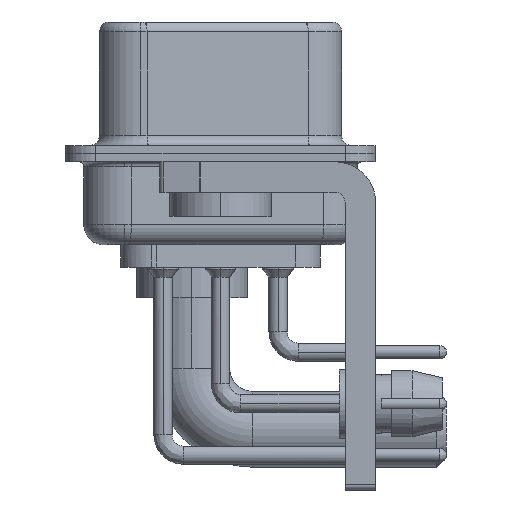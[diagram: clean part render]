
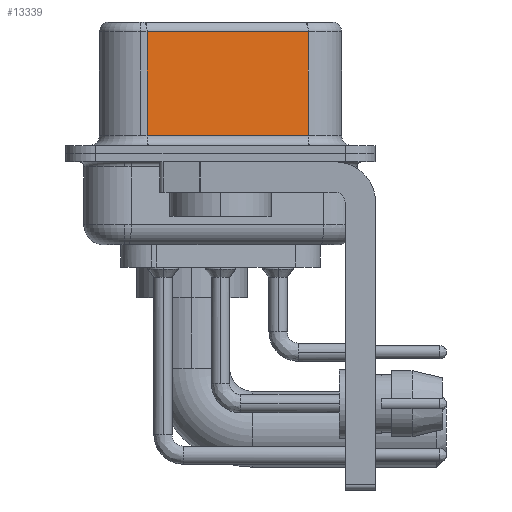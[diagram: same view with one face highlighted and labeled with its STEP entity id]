
A CAD part, left-side view. The second image highlights one B-rep face of the part: STEP entity #13339.
In plain terms, the highlighted planar face has unit normal (-0.985, -0.174, 0).
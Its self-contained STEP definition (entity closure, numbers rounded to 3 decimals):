
#404 = AXIS2_PLACEMENT_3D ( 'NONE', #25251, #5869, #31302 ) ;
#545 = PLANE ( 'NONE',  #404 ) ;
#2550 = CARTESIAN_POINT ( 'NONE',  ( 3.73, 3.628, 6.52 ) ) ;
#2779 = EDGE_LOOP ( 'NONE', ( #37489, #9758, #4748, #27221 ) ) ;
#4337 = EDGE_CURVE ( 'NONE', #12516, #39267, #35794, .T. ) ;
#4381 = LINE ( 'NONE', #7809, #28007 ) ;
#4582 = DIRECTION ( 'NONE',  ( 0.174, -0.985, 0. ) ) ;
#4748 = ORIENTED_EDGE ( 'NONE', *, *, #17851, .T. ) ;
#4954 = CARTESIAN_POINT ( 'NONE',  ( 3.73, 3.628, 6.02 ) ) ;
#5657 = LINE ( 'NONE', #23875, #7018 ) ;
#5869 = DIRECTION ( 'NONE',  ( 0.985, 0.174, 0. ) ) ;
#7018 = VECTOR ( 'NONE', #30346, 1000. ) ;
#7809 = CARTESIAN_POINT ( 'NONE',  ( 5.132, -4.322, 0.9 ) ) ;
#8096 = CARTESIAN_POINT ( 'NONE',  ( 5.132, -4.322, 6.02 ) ) ;
#9613 = VERTEX_POINT ( 'NONE', #18219 ) ;
#9758 = ORIENTED_EDGE ( 'NONE', *, *, #4337, .T. ) ;
#10350 = EDGE_CURVE ( 'NONE', #9613, #20329, #4381, .T. ) ;
#12516 = VERTEX_POINT ( 'NONE', #27430 ) ;
#13339 = ADVANCED_FACE ( 'NONE', ( #24087 ), #545, .F. ) ;
#16778 = EDGE_CURVE ( 'NONE', #12516, #20329, #5657, .T. ) ;
#17851 = EDGE_CURVE ( 'NONE', #39267, #9613, #33669, .T. ) ;
#18219 = CARTESIAN_POINT ( 'NONE',  ( 3.73, 3.628, 0.9 ) ) ;
#20017 = VECTOR ( 'NONE', #24595, 1000. ) ;
#20329 = VERTEX_POINT ( 'NONE', #22159 ) ;
#22159 = CARTESIAN_POINT ( 'NONE',  ( 5.132, -4.322, 0.9 ) ) ;
#23875 = CARTESIAN_POINT ( 'NONE',  ( 5.132, -4.322, 6.52 ) ) ;
#24087 = FACE_OUTER_BOUND ( 'NONE', #2779, .T. ) ;
#24595 = DIRECTION ( 'NONE',  ( 0., 0., -1. ) ) ;
#25251 = CARTESIAN_POINT ( 'NONE',  ( 5.132, -4.322, 6.52 ) ) ;
#27221 = ORIENTED_EDGE ( 'NONE', *, *, #10350, .T. ) ;
#27430 = CARTESIAN_POINT ( 'NONE',  ( 5.132, -4.322, 6.02 ) ) ;
#28007 = VECTOR ( 'NONE', #4582, 1000. ) ;
#30346 = DIRECTION ( 'NONE',  ( 0., 0., -1. ) ) ;
#31302 = DIRECTION ( 'NONE',  ( -0.174, 0.985, 0. ) ) ;
#33669 = LINE ( 'NONE', #2550, #20017 ) ;
#35168 = VECTOR ( 'NONE', #39045, 1000. ) ;
#35794 = LINE ( 'NONE', #8096, #35168 ) ;
#37489 = ORIENTED_EDGE ( 'NONE', *, *, #16778, .F. ) ;
#39045 = DIRECTION ( 'NONE',  ( -0.174, 0.985, 0. ) ) ;
#39267 = VERTEX_POINT ( 'NONE', #4954 ) ;
